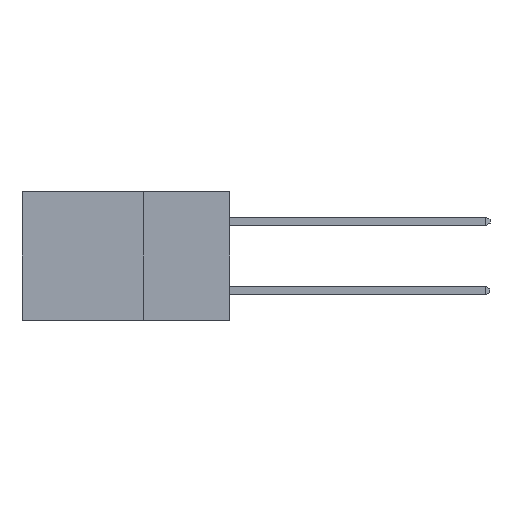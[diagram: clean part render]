
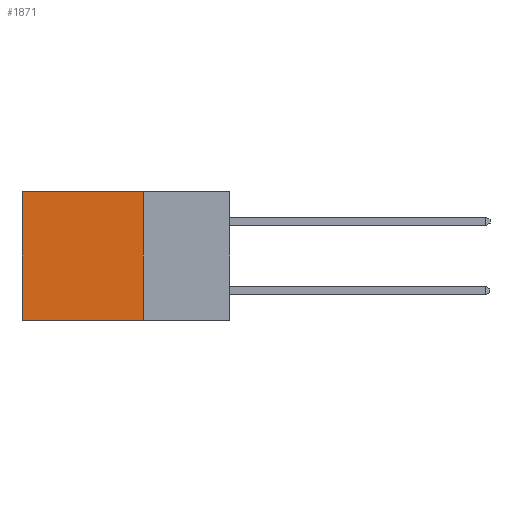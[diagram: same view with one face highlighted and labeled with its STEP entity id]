
A CAD part, left-side view. The second image highlights one B-rep face of the part: STEP entity #1871.
In plain terms, the highlighted planar face has unit normal (-1, 0, 0).
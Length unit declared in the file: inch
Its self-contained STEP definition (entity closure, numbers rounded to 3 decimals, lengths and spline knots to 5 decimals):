
#736 = LINE ( 'NONE', #16482, #8538 ) ;
#1077 = AXIS2_PLACEMENT_3D ( 'NONE', #3700, #9312, #9169 ) ;
#1871 = ADVANCED_FACE ( 'NONE', ( #3987 ), #6414, .F. ) ;
#2427 = EDGE_LOOP ( 'NONE', ( #4602, #6475, #4226, #7894 ) ) ;
#3096 = VERTEX_POINT ( 'NONE', #16565 ) ;
#3614 = EDGE_CURVE ( 'NONE', #19723, #14912, #736, .T. ) ;
#3700 = CARTESIAN_POINT ( 'NONE',  ( 0.298, 0.25, 0. ) ) ;
#3987 = FACE_OUTER_BOUND ( 'NONE', #2427, .T. ) ;
#4223 = EDGE_CURVE ( 'NONE', #14912, #3096, #18935, .T. ) ;
#4226 = ORIENTED_EDGE ( 'NONE', *, *, #3614, .F. ) ;
#4602 = ORIENTED_EDGE ( 'NONE', *, *, #18441, .T. ) ;
#4799 = DIRECTION ( 'NONE',  ( 0., 0., -1. ) ) ;
#6414 = PLANE ( 'NONE',  #1077 ) ;
#6445 = VECTOR ( 'NONE', #12478, 39.37008 ) ;
#6475 = ORIENTED_EDGE ( 'NONE', *, *, #4223, .F. ) ;
#7199 = CARTESIAN_POINT ( 'NONE',  ( 0.298, 0.25, 0. ) ) ;
#7629 = VECTOR ( 'NONE', #8700, 39.37008 ) ;
#7894 = ORIENTED_EDGE ( 'NONE', *, *, #18122, .T. ) ;
#8538 = VECTOR ( 'NONE', #17020, 39.37008 ) ;
#8700 = DIRECTION ( 'NONE',  ( 0., 1., 0. ) ) ;
#9169 = DIRECTION ( 'NONE',  ( 0., 0., -1. ) ) ;
#9312 = DIRECTION ( 'NONE',  ( 1., 0., 0. ) ) ;
#10068 = VECTOR ( 'NONE', #4799, 39.37008 ) ;
#10541 = LINE ( 'NONE', #14189, #10068 ) ;
#12228 = VERTEX_POINT ( 'NONE', #16991 ) ;
#12478 = DIRECTION ( 'NONE',  ( 0., 1., 0. ) ) ;
#14189 = CARTESIAN_POINT ( 'NONE',  ( 0.298, 0.6, 0. ) ) ;
#14912 = VERTEX_POINT ( 'NONE', #17540 ) ;
#14950 = CARTESIAN_POINT ( 'NONE',  ( 0.298, 0.25, -0.37 ) ) ;
#15994 = LINE ( 'NONE', #7199, #7629 ) ;
#16482 = CARTESIAN_POINT ( 'NONE',  ( 0.298, 0.25, 0. ) ) ;
#16565 = CARTESIAN_POINT ( 'NONE',  ( 0.298, 0.6, -0.37 ) ) ;
#16991 = CARTESIAN_POINT ( 'NONE',  ( 0.298, 0.6, 0. ) ) ;
#17020 = DIRECTION ( 'NONE',  ( 0., 0., -1. ) ) ;
#17540 = CARTESIAN_POINT ( 'NONE',  ( 0.298, 0.25, -0.37 ) ) ;
#18122 = EDGE_CURVE ( 'NONE', #19723, #12228, #15994, .T. ) ;
#18441 = EDGE_CURVE ( 'NONE', #12228, #3096, #10541, .T. ) ;
#18726 = CARTESIAN_POINT ( 'NONE',  ( 0.298, 0.25, 0. ) ) ;
#18935 = LINE ( 'NONE', #14950, #6445 ) ;
#19723 = VERTEX_POINT ( 'NONE', #18726 ) ;
